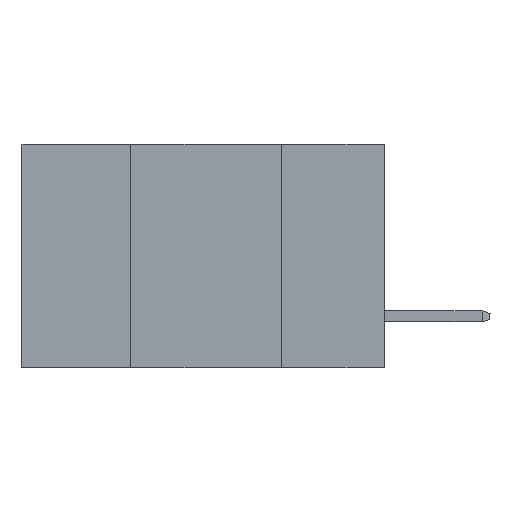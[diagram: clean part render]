
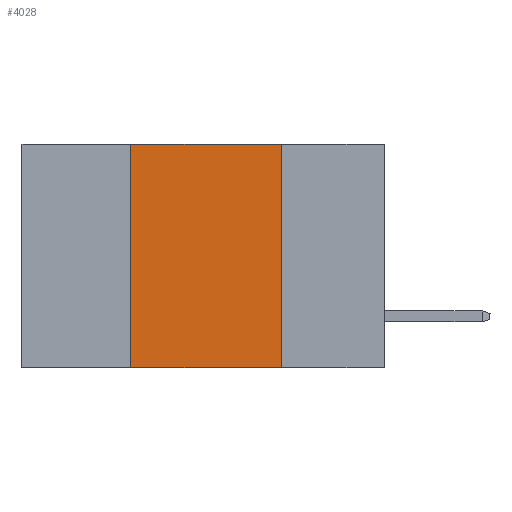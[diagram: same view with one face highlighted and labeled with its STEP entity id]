
A CAD part, left-side view. The second image highlights one B-rep face of the part: STEP entity #4028.
In plain terms, the highlighted planar face has unit normal (-1, 0, 0).
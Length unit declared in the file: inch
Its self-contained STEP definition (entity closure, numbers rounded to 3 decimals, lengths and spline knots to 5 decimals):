
#153 = EDGE_CURVE ( 'NONE', #9557, #7831, #3859, .T. ) ;
#1492 = ORIENTED_EDGE ( 'NONE', *, *, #1925, .F. ) ;
#1925 = EDGE_CURVE ( 'NONE', #7831, #3470, #2787, .T. ) ;
#2045 = VECTOR ( 'NONE', #10498, 39.37008 ) ;
#2214 = DIRECTION ( 'NONE',  ( 0., -1., 0. ) ) ;
#2434 = CARTESIAN_POINT ( 'NONE',  ( 0., 0.6, -0.37 ) ) ;
#2534 = EDGE_CURVE ( 'NONE', #2980, #3470, #7246, .T. ) ;
#2787 = LINE ( 'NONE', #6036, #3239 ) ;
#2980 = VERTEX_POINT ( 'NONE', #4812 ) ;
#3112 = CARTESIAN_POINT ( 'NONE',  ( 0., 0.17, -0.37 ) ) ;
#3239 = VECTOR ( 'NONE', #4245, 39.37008 ) ;
#3470 = VERTEX_POINT ( 'NONE', #3112 ) ;
#3859 = LINE ( 'NONE', #3909, #8066 ) ;
#3909 = CARTESIAN_POINT ( 'NONE',  ( 0., 0.6, 0. ) ) ;
#4000 = ORIENTED_EDGE ( 'NONE', *, *, #8645, .F. ) ;
#4028 = ADVANCED_FACE ( 'NONE', ( #5896 ), #6646, .F. ) ;
#4059 = EDGE_LOOP ( 'NONE', ( #1492, #5950, #4000, #7096 ) ) ;
#4245 = DIRECTION ( 'NONE',  ( 0., 0., -1. ) ) ;
#4663 = CARTESIAN_POINT ( 'NONE',  ( 0., 0.17, 0. ) ) ;
#4812 = CARTESIAN_POINT ( 'NONE',  ( 0., 0.42, -0.37 ) ) ;
#5547 = CARTESIAN_POINT ( 'NONE',  ( 0., 0.42, -0.37 ) ) ;
#5839 = CARTESIAN_POINT ( 'NONE',  ( 0., 0.6, 0. ) ) ;
#5870 = CARTESIAN_POINT ( 'NONE',  ( 0., 0.42, 0. ) ) ;
#5896 = FACE_OUTER_BOUND ( 'NONE', #4059, .T. ) ;
#5950 = ORIENTED_EDGE ( 'NONE', *, *, #153, .F. ) ;
#6036 = CARTESIAN_POINT ( 'NONE',  ( 0., 0.17, -0.37 ) ) ;
#6438 = AXIS2_PLACEMENT_3D ( 'NONE', #5839, #9921, #7448 ) ;
#6646 = PLANE ( 'NONE',  #6438 ) ;
#7096 = ORIENTED_EDGE ( 'NONE', *, *, #2534, .T. ) ;
#7246 = LINE ( 'NONE', #2434, #7551 ) ;
#7448 = DIRECTION ( 'NONE',  ( 0., 0., -1. ) ) ;
#7551 = VECTOR ( 'NONE', #8051, 39.37008 ) ;
#7831 = VERTEX_POINT ( 'NONE', #4663 ) ;
#8051 = DIRECTION ( 'NONE',  ( 0., -1., 0. ) ) ;
#8066 = VECTOR ( 'NONE', #2214, 39.37008 ) ;
#8645 = EDGE_CURVE ( 'NONE', #2980, #9557, #8816, .T. ) ;
#8816 = LINE ( 'NONE', #5547, #2045 ) ;
#9557 = VERTEX_POINT ( 'NONE', #5870 ) ;
#9921 = DIRECTION ( 'NONE',  ( 1., 0., 0. ) ) ;
#10498 = DIRECTION ( 'NONE',  ( 0., 0., 1. ) ) ;
